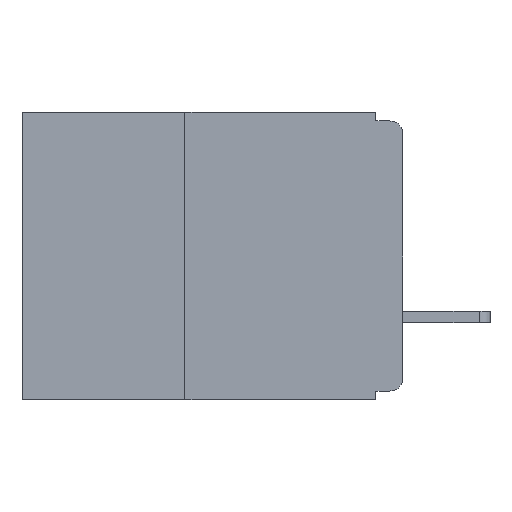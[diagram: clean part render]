
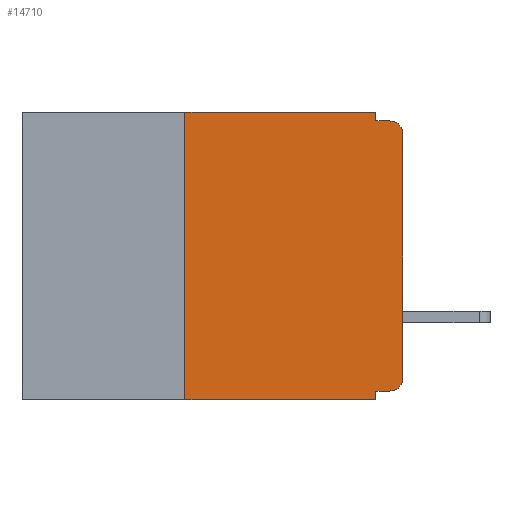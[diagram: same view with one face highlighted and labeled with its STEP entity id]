
A CAD part, left-side view. The second image highlights one B-rep face of the part: STEP entity #14710.
In plain terms, the highlighted planar face has unit normal (-1, 0, 0).
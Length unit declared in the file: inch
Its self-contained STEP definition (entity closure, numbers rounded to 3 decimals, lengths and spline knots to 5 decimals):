
#154 = VECTOR ( 'NONE', #12329, 39.37008 ) ;
#251 = ORIENTED_EDGE ( 'NONE', *, *, #26917, .F. ) ;
#656 = CARTESIAN_POINT ( 'NONE',  ( 0., 0.031, -0.33 ) ) ;
#1042 = EDGE_CURVE ( 'NONE', #16517, #19311, #23343, .T. ) ;
#1063 = EDGE_CURVE ( 'NONE', #9166, #18671, #29065, .T. ) ;
#1121 = ORIENTED_EDGE ( 'NONE', *, *, #26988, .F. ) ;
#1400 = VERTEX_POINT ( 'NONE', #19202 ) ;
#1696 = DIRECTION ( 'NONE',  ( 0., 0., -1. ) ) ;
#1883 = CARTESIAN_POINT ( 'NONE',  ( 0., 0.015, -0.01 ) ) ;
#2500 = CARTESIAN_POINT ( 'NONE',  ( 0., 0.437, 0. ) ) ;
#3592 = DIRECTION ( 'NONE',  ( -1., 0., 0. ) ) ;
#3667 = VECTOR ( 'NONE', #26641, 39.37008 ) ;
#4930 = ORIENTED_EDGE ( 'NONE', *, *, #14513, .T. ) ;
#5077 = VECTOR ( 'NONE', #29923, 39.37008 ) ;
#5481 = CARTESIAN_POINT ( 'NONE',  ( 0., 0.015, -0.32 ) ) ;
#5593 = ORIENTED_EDGE ( 'NONE', *, *, #1042, .T. ) ;
#5675 = EDGE_CURVE ( 'NONE', #8496, #23892, #24763, .T. ) ;
#6088 = CARTESIAN_POINT ( 'NONE',  ( 0., 0., -0.01 ) ) ;
#6264 = ORIENTED_EDGE ( 'NONE', *, *, #20015, .F. ) ;
#6473 = CARTESIAN_POINT ( 'NONE',  ( 0., 0., -0.305 ) ) ;
#6917 = CARTESIAN_POINT ( 'NONE',  ( 0., 0.437, 0. ) ) ;
#7049 = ORIENTED_EDGE ( 'NONE', *, *, #30250, .T. ) ;
#7344 = VECTOR ( 'NONE', #17841, 39.37008 ) ;
#7660 = AXIS2_PLACEMENT_3D ( 'NONE', #6917, #24158, #9430 ) ;
#7692 = VECTOR ( 'NONE', #8714, 39.37008 ) ;
#8281 = AXIS2_PLACEMENT_3D ( 'NONE', #18363, #3592, #20822 ) ;
#8326 = VECTOR ( 'NONE', #26822, 39.37008 ) ;
#8470 = LINE ( 'NONE', #6088, #7692 ) ;
#8496 = VERTEX_POINT ( 'NONE', #17994 ) ;
#8674 = FACE_OUTER_BOUND ( 'NONE', #25896, .T. ) ;
#8714 = DIRECTION ( 'NONE',  ( 0., -1., 0. ) ) ;
#9061 = VECTOR ( 'NONE', #14576, 39.37008 ) ;
#9166 = VERTEX_POINT ( 'NONE', #13156 ) ;
#9430 = DIRECTION ( 'NONE',  ( 0., 0., -1. ) ) ;
#9760 = CARTESIAN_POINT ( 'NONE',  ( 0., 0.25, -0.33 ) ) ;
#10027 = EDGE_CURVE ( 'NONE', #8496, #22091, #20633, .T. ) ;
#10651 = CIRCLE ( 'NONE', #8281, 0.015 ) ;
#10849 = ORIENTED_EDGE ( 'NONE', *, *, #1063, .F. ) ;
#11360 = EDGE_CURVE ( 'NONE', #1400, #23892, #13925, .T. ) ;
#11555 = ORIENTED_EDGE ( 'NONE', *, *, #10027, .F. ) ;
#12130 = ORIENTED_EDGE ( 'NONE', *, *, #11360, .F. ) ;
#12329 = DIRECTION ( 'NONE',  ( 0., -1., 0. ) ) ;
#13156 = CARTESIAN_POINT ( 'NONE',  ( 0., 0.031, 0. ) ) ;
#13327 = LINE ( 'NONE', #2500, #154 ) ;
#13925 = LINE ( 'NONE', #27622, #7344 ) ;
#14513 = EDGE_CURVE ( 'NONE', #26531, #16517, #10651, .T. ) ;
#14576 = DIRECTION ( 'NONE',  ( 0., 1., 0. ) ) ;
#14710 = ADVANCED_FACE ( 'NONE', ( #8674 ), #28960, .F. ) ;
#16461 = DIRECTION ( 'NONE',  ( -1., 0., 0. ) ) ;
#16517 = VERTEX_POINT ( 'NONE', #6473 ) ;
#17841 = DIRECTION ( 'NONE',  ( 0., 0., -1. ) ) ;
#17994 = CARTESIAN_POINT ( 'NONE',  ( 0., 0.25, -0.33 ) ) ;
#18104 = CARTESIAN_POINT ( 'NONE',  ( 0., 0.25, 0. ) ) ;
#18363 = CARTESIAN_POINT ( 'NONE',  ( 0., 0.015, -0.305 ) ) ;
#18671 = VERTEX_POINT ( 'NONE', #27826 ) ;
#19202 = CARTESIAN_POINT ( 'NONE',  ( 0., 0.031, -0.32 ) ) ;
#19311 = VERTEX_POINT ( 'NONE', #20567 ) ;
#20015 = EDGE_CURVE ( 'NONE', #18671, #22972, #8470, .T. ) ;
#20187 = CARTESIAN_POINT ( 'NONE',  ( 0., 0.437, -0.33 ) ) ;
#20268 = CARTESIAN_POINT ( 'NONE',  ( 0., 0., 0. ) ) ;
#20324 = DIRECTION ( 'NONE',  ( 0., 0., -1. ) ) ;
#20567 = CARTESIAN_POINT ( 'NONE',  ( 0., 0., -0.025 ) ) ;
#20633 = LINE ( 'NONE', #9760, #8326 ) ;
#20822 = DIRECTION ( 'NONE',  ( 0., 0., -1. ) ) ;
#21861 = CARTESIAN_POINT ( 'NONE',  ( 0., 0., -0.32 ) ) ;
#22091 = VERTEX_POINT ( 'NONE', #18104 ) ;
#22131 = LINE ( 'NONE', #21861, #9061 ) ;
#22972 = VERTEX_POINT ( 'NONE', #1883 ) ;
#23343 = LINE ( 'NONE', #20268, #3667 ) ;
#23892 = VERTEX_POINT ( 'NONE', #656 ) ;
#24109 = VECTOR ( 'NONE', #20324, 39.37008 ) ;
#24158 = DIRECTION ( 'NONE',  ( 1., 0., 0. ) ) ;
#24763 = LINE ( 'NONE', #20187, #5077 ) ;
#25038 = AXIS2_PLACEMENT_3D ( 'NONE', #31127, #16461, #1696 ) ;
#25675 = CIRCLE ( 'NONE', #25038, 0.015 ) ;
#25896 = EDGE_LOOP ( 'NONE', ( #5593, #7049, #6264, #10849, #1121, #11555, #29400, #12130, #251, #4930 ) ) ;
#26531 = VERTEX_POINT ( 'NONE', #5481 ) ;
#26641 = DIRECTION ( 'NONE',  ( 0., 0., 1. ) ) ;
#26822 = DIRECTION ( 'NONE',  ( 0., 0., 1. ) ) ;
#26917 = EDGE_CURVE ( 'NONE', #26531, #1400, #22131, .T. ) ;
#26988 = EDGE_CURVE ( 'NONE', #22091, #9166, #13327, .T. ) ;
#27622 = CARTESIAN_POINT ( 'NONE',  ( 0., 0.031, -0.33 ) ) ;
#27826 = CARTESIAN_POINT ( 'NONE',  ( 0., 0.031, -0.01 ) ) ;
#28960 = PLANE ( 'NONE',  #7660 ) ;
#29065 = LINE ( 'NONE', #29274, #24109 ) ;
#29274 = CARTESIAN_POINT ( 'NONE',  ( 0., 0.031, 0. ) ) ;
#29400 = ORIENTED_EDGE ( 'NONE', *, *, #5675, .T. ) ;
#29923 = DIRECTION ( 'NONE',  ( 0., -1., 0. ) ) ;
#30250 = EDGE_CURVE ( 'NONE', #19311, #22972, #25675, .T. ) ;
#31127 = CARTESIAN_POINT ( 'NONE',  ( 0., 0.015, -0.025 ) ) ;
